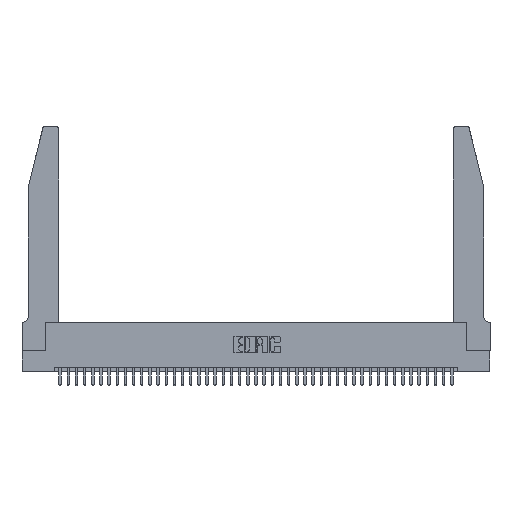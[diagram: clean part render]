
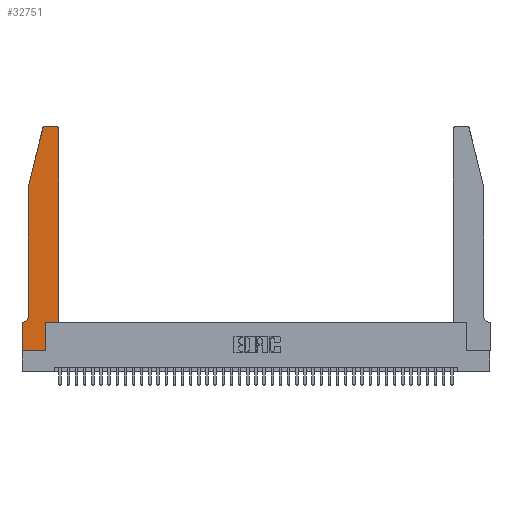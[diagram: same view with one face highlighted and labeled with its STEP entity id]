
A CAD part, top view. The second image highlights one B-rep face of the part: STEP entity #32751.
In plain terms, the highlighted planar face has unit normal (0, 0, 1).
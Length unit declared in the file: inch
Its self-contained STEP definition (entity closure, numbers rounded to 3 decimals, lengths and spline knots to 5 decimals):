
#51 = DIRECTION ( 'NONE',  ( 1., 0., 0. ) ) ;
#180 = CARTESIAN_POINT ( 'NONE',  ( 0., 0.35, 0.37 ) ) ;
#455 = ORIENTED_EDGE ( 'NONE', *, *, #3665, .T. ) ;
#1772 = DIRECTION ( 'NONE',  ( 0., 0., -1. ) ) ;
#2206 = LINE ( 'NONE', #35153, #8860 ) ;
#3665 = EDGE_CURVE ( 'NONE', #14093, #8346, #9459, .T. ) ;
#3669 = CARTESIAN_POINT ( 'NONE',  ( 0.0055, 0.42, 0.37 ) ) ;
#3678 = VECTOR ( 'NONE', #22291, 39.37008 ) ;
#3723 = ORIENTED_EDGE ( 'NONE', *, *, #28512, .T. ) ;
#4018 = EDGE_CURVE ( 'NONE', #20225, #25298, #11435, .T. ) ;
#4120 = DIRECTION ( 'NONE',  ( 0., 0., 1. ) ) ;
#4479 = AXIS2_PLACEMENT_3D ( 'NONE', #3669, #1772, #30243 ) ;
#4660 = AXIS2_PLACEMENT_3D ( 'NONE', #23737, #4120, #10704 ) ;
#4885 = ORIENTED_EDGE ( 'NONE', *, *, #10050, .T. ) ;
#5777 = CARTESIAN_POINT ( 'NONE',  ( 0., 0.35, 0.37 ) ) ;
#5792 = CARTESIAN_POINT ( 'NONE',  ( 0.4505, 2.72, 0.37 ) ) ;
#6463 = VECTOR ( 'NONE', #6540, 39.37008 ) ;
#6540 = DIRECTION ( 'NONE',  ( 0., 1., 0. ) ) ;
#7219 = ORIENTED_EDGE ( 'NONE', *, *, #40421, .T. ) ;
#8346 = VERTEX_POINT ( 'NONE', #40482 ) ;
#8596 = ORIENTED_EDGE ( 'NONE', *, *, #38418, .T. ) ;
#8768 = AXIS2_PLACEMENT_3D ( 'NONE', #27734, #14664, #21277 ) ;
#8860 = VECTOR ( 'NONE', #38720, 39.37008 ) ;
#9044 = ORIENTED_EDGE ( 'NONE', *, *, #17601, .T. ) ;
#9459 = LINE ( 'NONE', #39850, #29968 ) ;
#9684 = ORIENTED_EDGE ( 'NONE', *, *, #11405, .T. ) ;
#9878 = VECTOR ( 'NONE', #18456, 39.37008 ) ;
#10050 = EDGE_CURVE ( 'NONE', #28064, #40798, #34825, .T. ) ;
#10220 = DIRECTION ( 'NONE',  ( 0., 0., 1. ) ) ;
#10704 = DIRECTION ( 'NONE',  ( 1., 0., 0. ) ) ;
#11405 = EDGE_CURVE ( 'NONE', #20430, #14093, #21907, .T. ) ;
#11435 = CIRCLE ( 'NONE', #4479, 0.07 ) ;
#13276 = ORIENTED_EDGE ( 'NONE', *, *, #4018, .T. ) ;
#13385 = LINE ( 'NONE', #19020, #3678 ) ;
#14093 = VERTEX_POINT ( 'NONE', #19073 ) ;
#14329 = VERTEX_POINT ( 'NONE', #29908 ) ;
#14664 = DIRECTION ( 'NONE',  ( 0., 0., 1. ) ) ;
#16728 = CARTESIAN_POINT ( 'NONE',  ( 0.0755, 2., 0.37 ) ) ;
#16913 = CIRCLE ( 'NONE', #8768, 0.03 ) ;
#17601 = EDGE_CURVE ( 'NONE', #33108, #40388, #39082, .T. ) ;
#17875 = EDGE_CURVE ( 'NONE', #40388, #28064, #2206, .T. ) ;
#18251 = VECTOR ( 'NONE', #39632, 39.37008 ) ;
#18375 = EDGE_CURVE ( 'NONE', #25298, #33108, #20078, .T. ) ;
#18456 = DIRECTION ( 'NONE',  ( 0., -1., 0. ) ) ;
#18717 = EDGE_CURVE ( 'NONE', #14329, #20430, #37655, .T. ) ;
#19020 = CARTESIAN_POINT ( 'NONE',  ( 0.0755, 2., 0.37 ) ) ;
#19073 = CARTESIAN_POINT ( 'NONE',  ( 0.4205, 2.75, 0.37 ) ) ;
#19494 = DIRECTION ( 'NONE',  ( -1., 0., 0. ) ) ;
#20078 = LINE ( 'NONE', #25520, #23143 ) ;
#20225 = VERTEX_POINT ( 'NONE', #39592 ) ;
#20430 = VERTEX_POINT ( 'NONE', #5792 ) ;
#20583 = DIRECTION ( 'NONE',  ( -1., 0., 0. ) ) ;
#20591 = DIRECTION ( 'NONE',  ( 0., 1., 0. ) ) ;
#21277 = DIRECTION ( 'NONE',  ( 1., 0., 0. ) ) ;
#21860 = EDGE_LOOP ( 'NONE', ( #455, #8596, #3723, #7219, #13276, #27589, #9044, #37784, #4885, #25754, #39158, #9684 ) ) ;
#21907 = CIRCLE ( 'NONE', #4660, 0.03 ) ;
#22291 = DIRECTION ( 'NONE',  ( -0.239, -0.971, 0. ) ) ;
#22303 = CARTESIAN_POINT ( 'NONE',  ( 0.2865, 0.35, 0.37 ) ) ;
#23143 = VECTOR ( 'NONE', #19494, 39.37008 ) ;
#23430 = AXIS2_PLACEMENT_3D ( 'NONE', #180, #10220, #51 ) ;
#23737 = CARTESIAN_POINT ( 'NONE',  ( 0.4205, 2.72, 0.37 ) ) ;
#23893 = CARTESIAN_POINT ( 'NONE',  ( 0., 0., 0.37 ) ) ;
#24019 = FACE_OUTER_BOUND ( 'NONE', #21860, .T. ) ;
#25298 = VERTEX_POINT ( 'NONE', #40487 ) ;
#25520 = CARTESIAN_POINT ( 'NONE',  ( 0.0755, 0.35, 0.37 ) ) ;
#25754 = ORIENTED_EDGE ( 'NONE', *, *, #36620, .T. ) ;
#25956 = CARTESIAN_POINT ( 'NONE',  ( 0.2865, 0., 0.37 ) ) ;
#26629 = VECTOR ( 'NONE', #20591, 39.37008 ) ;
#27589 = ORIENTED_EDGE ( 'NONE', *, *, #18375, .T. ) ;
#27734 = CARTESIAN_POINT ( 'NONE',  ( 0.284, 2.72, 0.37 ) ) ;
#28064 = VERTEX_POINT ( 'NONE', #25956 ) ;
#28512 = EDGE_CURVE ( 'NONE', #29386, #37710, #13385, .T. ) ;
#29386 = VERTEX_POINT ( 'NONE', #33498 ) ;
#29487 = CARTESIAN_POINT ( 'NONE',  ( 0.4505, 0.35, 0.37 ) ) ;
#29611 = PLANE ( 'NONE',  #23430 ) ;
#29908 = CARTESIAN_POINT ( 'NONE',  ( 0.4505, 0.35, 0.37 ) ) ;
#29968 = VECTOR ( 'NONE', #20583, 39.37008 ) ;
#30243 = DIRECTION ( 'NONE',  ( -1., 0., 0. ) ) ;
#30876 = VECTOR ( 'NONE', #40990, 39.37008 ) ;
#31011 = CARTESIAN_POINT ( 'NONE',  ( 0.4505, 0.35, 0.37 ) ) ;
#32751 = ADVANCED_FACE ( 'NONE', ( #24019 ), #29611, .T. ) ;
#33108 = VERTEX_POINT ( 'NONE', #5777 ) ;
#33498 = CARTESIAN_POINT ( 'NONE',  ( 0.25487, 2.72718, 0.37 ) ) ;
#33902 = CARTESIAN_POINT ( 'NONE',  ( 0.0755, 2., 0.37 ) ) ;
#34825 = LINE ( 'NONE', #40134, #26629 ) ;
#35153 = CARTESIAN_POINT ( 'NONE',  ( 0., 0., 0.37 ) ) ;
#36620 = EDGE_CURVE ( 'NONE', #40798, #14329, #37493, .T. ) ;
#37493 = LINE ( 'NONE', #31011, #30876 ) ;
#37655 = LINE ( 'NONE', #29487, #6463 ) ;
#37710 = VERTEX_POINT ( 'NONE', #33902 ) ;
#37752 = CARTESIAN_POINT ( 'NONE',  ( 0., 0., 0.37 ) ) ;
#37784 = ORIENTED_EDGE ( 'NONE', *, *, #17875, .T. ) ;
#38418 = EDGE_CURVE ( 'NONE', #8346, #29386, #16913, .T. ) ;
#38720 = DIRECTION ( 'NONE',  ( 1., 0., 0. ) ) ;
#39082 = LINE ( 'NONE', #37752, #9878 ) ;
#39158 = ORIENTED_EDGE ( 'NONE', *, *, #18717, .T. ) ;
#39592 = CARTESIAN_POINT ( 'NONE',  ( 0.0755, 0.42, 0.37 ) ) ;
#39632 = DIRECTION ( 'NONE',  ( 0., -1., 0. ) ) ;
#39719 = LINE ( 'NONE', #16728, #18251 ) ;
#39850 = CARTESIAN_POINT ( 'NONE',  ( 0.2605, 2.75, 0.37 ) ) ;
#40134 = CARTESIAN_POINT ( 'NONE',  ( 0.2865, 0.35, 0.37 ) ) ;
#40388 = VERTEX_POINT ( 'NONE', #23893 ) ;
#40421 = EDGE_CURVE ( 'NONE', #37710, #20225, #39719, .T. ) ;
#40482 = CARTESIAN_POINT ( 'NONE',  ( 0.284, 2.75, 0.37 ) ) ;
#40487 = CARTESIAN_POINT ( 'NONE',  ( 0.0055, 0.35, 0.37 ) ) ;
#40798 = VERTEX_POINT ( 'NONE', #22303 ) ;
#40990 = DIRECTION ( 'NONE',  ( 1., 0., 0. ) ) ;
